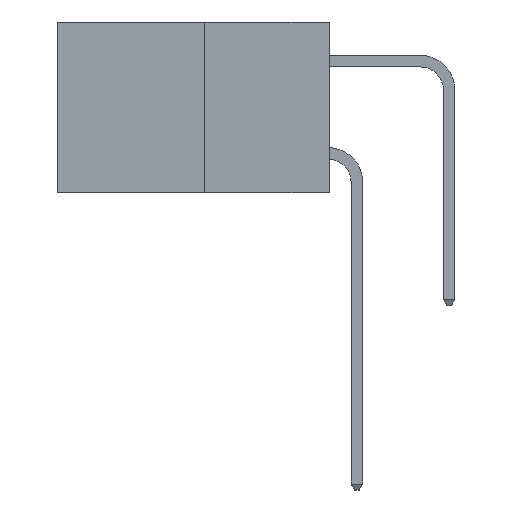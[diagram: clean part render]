
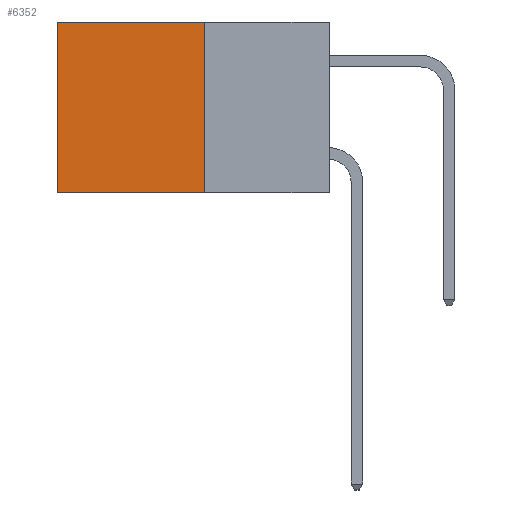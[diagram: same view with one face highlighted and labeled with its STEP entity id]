
A CAD part, left-side view. The second image highlights one B-rep face of the part: STEP entity #6352.
In plain terms, the highlighted planar face has unit normal (-1, 0, 0).
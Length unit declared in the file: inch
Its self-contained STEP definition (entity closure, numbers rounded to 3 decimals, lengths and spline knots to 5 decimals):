
#148 = ORIENTED_EDGE ( 'NONE', *, *, #6702, .T. ) ;
#178 = FACE_OUTER_BOUND ( 'NONE', #13969, .T. ) ;
#558 = VERTEX_POINT ( 'NONE', #3675 ) ;
#603 = LINE ( 'NONE', #9387, #12467 ) ;
#1122 = VECTOR ( 'NONE', #14657, 39.37008 ) ;
#1566 = VERTEX_POINT ( 'NONE', #13906 ) ;
#2167 = EDGE_CURVE ( 'NONE', #558, #1566, #9638, .T. ) ;
#2779 = DIRECTION ( 'NONE',  ( 0., 0., -1. ) ) ;
#2961 = CARTESIAN_POINT ( 'NONE',  ( 0.277, 0.27, 0. ) ) ;
#3675 = CARTESIAN_POINT ( 'NONE',  ( 0.277, 0.59, 0. ) ) ;
#3866 = CARTESIAN_POINT ( 'NONE',  ( 0.277, 0.27, -0.37 ) ) ;
#4817 = DIRECTION ( 'NONE',  ( 0., 0., -1. ) ) ;
#5256 = DIRECTION ( 'NONE',  ( 0., 1., 0. ) ) ;
#6021 = AXIS2_PLACEMENT_3D ( 'NONE', #3866, #9641, #2779 ) ;
#6352 = ADVANCED_FACE ( 'NONE', ( #178 ), #8476, .F. ) ;
#6702 = EDGE_CURVE ( 'NONE', #11226, #558, #13523, .T. ) ;
#6930 = VERTEX_POINT ( 'NONE', #12549 ) ;
#7233 = LINE ( 'NONE', #13478, #1122 ) ;
#8476 = PLANE ( 'NONE',  #6021 ) ;
#9246 = ORIENTED_EDGE ( 'NONE', *, *, #14585, .F. ) ;
#9387 = CARTESIAN_POINT ( 'NONE',  ( 0.277, 0.27, -0.37 ) ) ;
#9638 = LINE ( 'NONE', #13138, #9987 ) ;
#9641 = DIRECTION ( 'NONE',  ( 1., 0., 0. ) ) ;
#9987 = VECTOR ( 'NONE', #13056, 39.37008 ) ;
#10083 = EDGE_CURVE ( 'NONE', #6930, #1566, #7233, .T. ) ;
#10412 = VECTOR ( 'NONE', #5256, 39.37008 ) ;
#11226 = VERTEX_POINT ( 'NONE', #14364 ) ;
#12467 = VECTOR ( 'NONE', #4817, 39.37008 ) ;
#12511 = ORIENTED_EDGE ( 'NONE', *, *, #10083, .F. ) ;
#12549 = CARTESIAN_POINT ( 'NONE',  ( 0.277, 0.27, -0.37 ) ) ;
#13056 = DIRECTION ( 'NONE',  ( 0., 0., -1. ) ) ;
#13138 = CARTESIAN_POINT ( 'NONE',  ( 0.277, 0.59, -0.37 ) ) ;
#13478 = CARTESIAN_POINT ( 'NONE',  ( 0.277, 0.27, -0.37 ) ) ;
#13523 = LINE ( 'NONE', #2961, #10412 ) ;
#13906 = CARTESIAN_POINT ( 'NONE',  ( 0.277, 0.59, -0.37 ) ) ;
#13969 = EDGE_LOOP ( 'NONE', ( #14154, #12511, #9246, #148 ) ) ;
#14154 = ORIENTED_EDGE ( 'NONE', *, *, #2167, .T. ) ;
#14364 = CARTESIAN_POINT ( 'NONE',  ( 0.277, 0.27, 0. ) ) ;
#14585 = EDGE_CURVE ( 'NONE', #11226, #6930, #603, .T. ) ;
#14657 = DIRECTION ( 'NONE',  ( 0., 1., 0. ) ) ;
